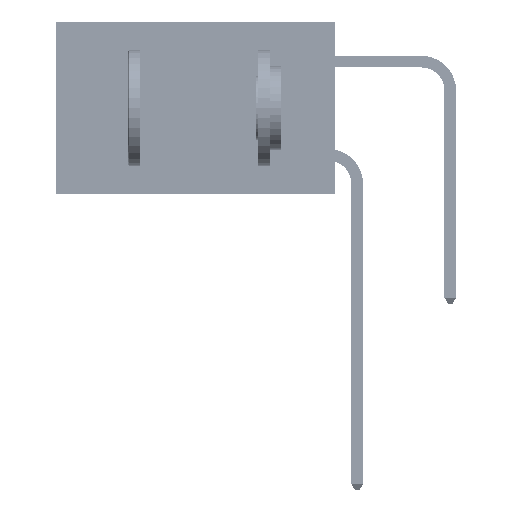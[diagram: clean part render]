
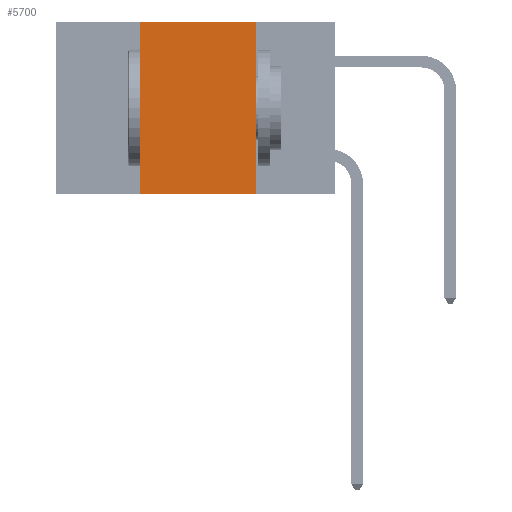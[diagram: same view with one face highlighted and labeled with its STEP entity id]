
A CAD part, left-side view. The second image highlights one B-rep face of the part: STEP entity #5700.
In plain terms, the highlighted planar face has unit normal (-1, 0, 0).
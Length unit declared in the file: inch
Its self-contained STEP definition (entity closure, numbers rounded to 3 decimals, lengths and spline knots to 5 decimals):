
#2833 = LINE ( 'NONE', #20220, #41953 ) ;
#5700 = ADVANCED_FACE ( 'NONE', ( #39975 ), #23589, .F. ) ;
#6989 = VERTEX_POINT ( 'NONE', #37834 ) ;
#7050 = VERTEX_POINT ( 'NONE', #45892 ) ;
#7987 = EDGE_CURVE ( 'NONE', #7050, #6989, #46835, .T. ) ;
#8089 = VECTOR ( 'NONE', #14235, 39.37008 ) ;
#9023 = EDGE_CURVE ( 'NONE', #7050, #9118, #2833, .T. ) ;
#9118 = VERTEX_POINT ( 'NONE', #28033 ) ;
#9651 = ORIENTED_EDGE ( 'NONE', *, *, #16896, .F. ) ;
#9733 = DIRECTION ( 'NONE',  ( 0., 0., 1. ) ) ;
#10107 = VECTOR ( 'NONE', #9733, 39.37008 ) ;
#12314 = CARTESIAN_POINT ( 'NONE',  ( 0., 0.6, 0. ) ) ;
#12984 = CARTESIAN_POINT ( 'NONE',  ( 0., 0.17, 0. ) ) ;
#13195 = VERTEX_POINT ( 'NONE', #12984 ) ;
#13800 = ORIENTED_EDGE ( 'NONE', *, *, #7987, .F. ) ;
#14235 = DIRECTION ( 'NONE',  ( 0., 0., -1. ) ) ;
#15847 = ORIENTED_EDGE ( 'NONE', *, *, #37975, .F. ) ;
#16617 = DIRECTION ( 'NONE',  ( 0., -1., 0. ) ) ;
#16896 = EDGE_CURVE ( 'NONE', #13195, #9118, #38341, .T. ) ;
#18155 = ORIENTED_EDGE ( 'NONE', *, *, #9023, .T. ) ;
#19930 = CARTESIAN_POINT ( 'NONE',  ( 0., 0.6, 0. ) ) ;
#20198 = VECTOR ( 'NONE', #16617, 39.37008 ) ;
#20220 = CARTESIAN_POINT ( 'NONE',  ( 0., 0.6, -0.37 ) ) ;
#23589 = PLANE ( 'NONE',  #45615 ) ;
#25003 = CARTESIAN_POINT ( 'NONE',  ( 0., 0.17, 0. ) ) ;
#28033 = CARTESIAN_POINT ( 'NONE',  ( 0., 0.17, -0.37 ) ) ;
#29654 = EDGE_LOOP ( 'NONE', ( #9651, #15847, #13800, #18155 ) ) ;
#32446 = CARTESIAN_POINT ( 'NONE',  ( 0., 0.42, 0. ) ) ;
#37834 = CARTESIAN_POINT ( 'NONE',  ( 0., 0.42, 0. ) ) ;
#37975 = EDGE_CURVE ( 'NONE', #6989, #13195, #39765, .T. ) ;
#38341 = LINE ( 'NONE', #25003, #8089 ) ;
#38526 = DIRECTION ( 'NONE',  ( 0., 0., -1. ) ) ;
#39765 = LINE ( 'NONE', #12314, #20198 ) ;
#39975 = FACE_OUTER_BOUND ( 'NONE', #29654, .T. ) ;
#41953 = VECTOR ( 'NONE', #43247, 39.37008 ) ;
#43247 = DIRECTION ( 'NONE',  ( 0., -1., 0. ) ) ;
#45615 = AXIS2_PLACEMENT_3D ( 'NONE', #19930, #46436, #38526 ) ;
#45892 = CARTESIAN_POINT ( 'NONE',  ( 0., 0.42, -0.37 ) ) ;
#46436 = DIRECTION ( 'NONE',  ( 1., 0., 0. ) ) ;
#46835 = LINE ( 'NONE', #32446, #10107 ) ;
